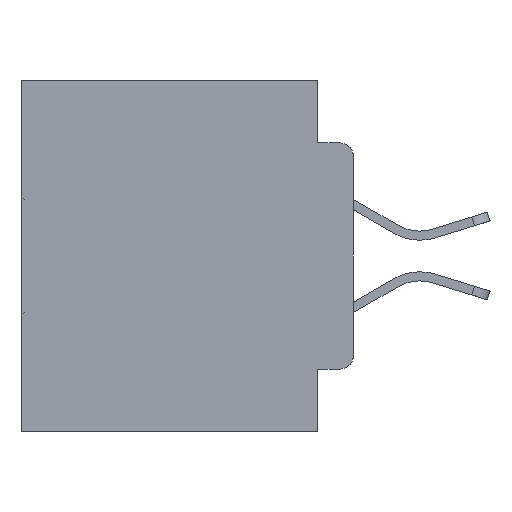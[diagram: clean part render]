
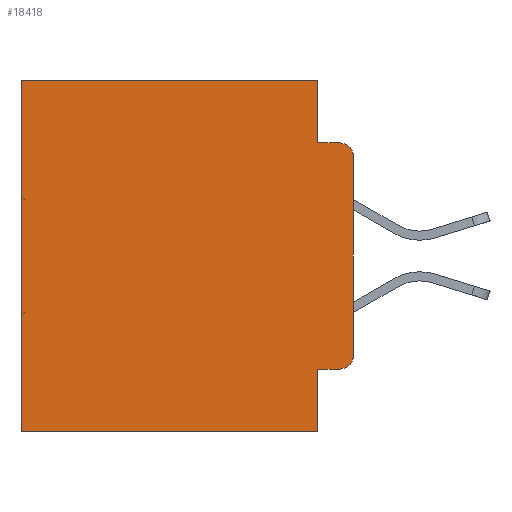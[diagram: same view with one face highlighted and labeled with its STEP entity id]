
A CAD part, left-side view. The second image highlights one B-rep face of the part: STEP entity #18418.
In plain terms, the highlighted planar face has unit normal (-1, 0, 0).
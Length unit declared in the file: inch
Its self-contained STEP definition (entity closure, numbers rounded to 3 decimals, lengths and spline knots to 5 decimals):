
#208 = CARTESIAN_POINT ( 'NONE',  ( 0.298, 0.473, 0. ) ) ;
#493 = CARTESIAN_POINT ( 'NONE',  ( 0.298, 0.051, 0. ) ) ;
#1325 = CARTESIAN_POINT ( 'NONE',  ( 0.298, 0.051, -0.0885 ) ) ;
#1453 = CARTESIAN_POINT ( 'NONE',  ( 0.298, 0.051, 0. ) ) ;
#1546 = VERTEX_POINT ( 'NONE', #14680 ) ;
#1714 = EDGE_CURVE ( 'NONE', #9751, #1546, #14060, .T. ) ;
#2243 = LINE ( 'NONE', #13286, #20582 ) ;
#2251 = LINE ( 'NONE', #27354, #27977 ) ;
#2500 = CARTESIAN_POINT ( 'NONE',  ( 0.298, 0.051, -0.4115 ) ) ;
#2796 = CARTESIAN_POINT ( 'NONE',  ( 0.298, 0.473, -0.5 ) ) ;
#2887 = CARTESIAN_POINT ( 'NONE',  ( 0.298, 0.051, 0. ) ) ;
#3196 = EDGE_CURVE ( 'NONE', #13413, #29406, #16702, .T. ) ;
#3842 = CARTESIAN_POINT ( 'NONE',  ( 0.298, 0.473, 0. ) ) ;
#3933 = DIRECTION ( 'NONE',  ( 0., 0., -1. ) ) ;
#5208 = DIRECTION ( 'NONE',  ( 0., -1., 0. ) ) ;
#7152 = DIRECTION ( 'NONE',  ( -1., 0., 0. ) ) ;
#7243 = VERTEX_POINT ( 'NONE', #1453 ) ;
#7281 = DIRECTION ( 'NONE',  ( 1., 0., 0. ) ) ;
#7400 = DIRECTION ( 'NONE',  ( 0., 0., -1. ) ) ;
#7687 = EDGE_CURVE ( 'NONE', #7243, #22381, #15127, .T. ) ;
#9164 = ORIENTED_EDGE ( 'NONE', *, *, #30143, .T. ) ;
#9751 = VERTEX_POINT ( 'NONE', #31680 ) ;
#10333 = EDGE_CURVE ( 'NONE', #22381, #19065, #28598, .T. ) ;
#13094 = VERTEX_POINT ( 'NONE', #1325 ) ;
#13286 = CARTESIAN_POINT ( 'NONE',  ( 0.298, 0.051, -0.0885 ) ) ;
#13410 = EDGE_CURVE ( 'NONE', #9751, #15226, #2251, .T. ) ;
#13413 = VERTEX_POINT ( 'NONE', #2500 ) ;
#13834 = CARTESIAN_POINT ( 'NONE',  ( 0.298, 0., -0.3915 ) ) ;
#14060 = CIRCLE ( 'NONE', #30863, 0.02 ) ;
#14680 = CARTESIAN_POINT ( 'NONE',  ( 0.298, 0.02, -0.0885 ) ) ;
#15127 = LINE ( 'NONE', #32003, #20955 ) ;
#15196 = FACE_OUTER_BOUND ( 'NONE', #16358, .T. ) ;
#15226 = VERTEX_POINT ( 'NONE', #13834 ) ;
#16358 = EDGE_LOOP ( 'NONE', ( #20195, #21744, #18322, #17511, #27207, #32156, #25284, #31083, #28011, #9164 ) ) ;
#16619 = LINE ( 'NONE', #493, #29809 ) ;
#16702 = LINE ( 'NONE', #17954, #22491 ) ;
#16835 = LINE ( 'NONE', #2887, #22619 ) ;
#17296 = CARTESIAN_POINT ( 'NONE',  ( 0.298, 0., -0.5 ) ) ;
#17442 = EDGE_CURVE ( 'NONE', #13413, #28976, #16835, .T. ) ;
#17511 = ORIENTED_EDGE ( 'NONE', *, *, #27279, .F. ) ;
#17954 = CARTESIAN_POINT ( 'NONE',  ( 0.298, 0.051, -0.4115 ) ) ;
#18322 = ORIENTED_EDGE ( 'NONE', *, *, #26248, .F. ) ;
#18418 = ADVANCED_FACE ( 'NONE', ( #15196 ), #27150, .F. ) ;
#19065 = VERTEX_POINT ( 'NONE', #2796 ) ;
#19642 = CARTESIAN_POINT ( 'NONE',  ( 0.298, 0., 0. ) ) ;
#20195 = ORIENTED_EDGE ( 'NONE', *, *, #13410, .F. ) ;
#20582 = VECTOR ( 'NONE', #23174, 39.37008 ) ;
#20920 = AXIS2_PLACEMENT_3D ( 'NONE', #19642, #7281, #24743 ) ;
#20955 = VECTOR ( 'NONE', #21054, 39.37008 ) ;
#21054 = DIRECTION ( 'NONE',  ( 0., 1., 0. ) ) ;
#21621 = EDGE_CURVE ( 'NONE', #28976, #19065, #28153, .T. ) ;
#21744 = ORIENTED_EDGE ( 'NONE', *, *, #1714, .T. ) ;
#21951 = VECTOR ( 'NONE', #3933, 39.37008 ) ;
#22078 = CARTESIAN_POINT ( 'NONE',  ( 0.298, 0.02, -0.3915 ) ) ;
#22274 = VECTOR ( 'NONE', #32058, 39.37008 ) ;
#22381 = VERTEX_POINT ( 'NONE', #208 ) ;
#22487 = CARTESIAN_POINT ( 'NONE',  ( 0.298, 0.051, -0.5 ) ) ;
#22491 = VECTOR ( 'NONE', #5208, 39.37008 ) ;
#22619 = VECTOR ( 'NONE', #22825, 39.37008 ) ;
#22825 = DIRECTION ( 'NONE',  ( 0., 0., -1. ) ) ;
#23174 = DIRECTION ( 'NONE',  ( 0., -1., 0. ) ) ;
#23420 = CIRCLE ( 'NONE', #32046, 0.02 ) ;
#24620 = DIRECTION ( 'NONE',  ( 0., 0., -1. ) ) ;
#24743 = DIRECTION ( 'NONE',  ( 0., 0., -1. ) ) ;
#25284 = ORIENTED_EDGE ( 'NONE', *, *, #21621, .F. ) ;
#25457 = DIRECTION ( 'NONE',  ( 0., 0., -1. ) ) ;
#26061 = DIRECTION ( 'NONE',  ( -1., 0., 0. ) ) ;
#26248 = EDGE_CURVE ( 'NONE', #13094, #1546, #2243, .T. ) ;
#26312 = CARTESIAN_POINT ( 'NONE',  ( 0.298, 0.02, -0.4115 ) ) ;
#27150 = PLANE ( 'NONE',  #20920 ) ;
#27207 = ORIENTED_EDGE ( 'NONE', *, *, #7687, .T. ) ;
#27279 = EDGE_CURVE ( 'NONE', #7243, #13094, #16619, .T. ) ;
#27354 = CARTESIAN_POINT ( 'NONE',  ( 0.298, 0., 0. ) ) ;
#27977 = VECTOR ( 'NONE', #7400, 39.37008 ) ;
#28011 = ORIENTED_EDGE ( 'NONE', *, *, #3196, .T. ) ;
#28153 = LINE ( 'NONE', #17296, #22274 ) ;
#28598 = LINE ( 'NONE', #3842, #21951 ) ;
#28976 = VERTEX_POINT ( 'NONE', #22487 ) ;
#29300 = DIRECTION ( 'NONE',  ( 0., 0., -1. ) ) ;
#29406 = VERTEX_POINT ( 'NONE', #26312 ) ;
#29809 = VECTOR ( 'NONE', #25457, 39.37008 ) ;
#30143 = EDGE_CURVE ( 'NONE', #29406, #15226, #23420, .T. ) ;
#30863 = AXIS2_PLACEMENT_3D ( 'NONE', #31838, #26061, #29300 ) ;
#31083 = ORIENTED_EDGE ( 'NONE', *, *, #17442, .F. ) ;
#31680 = CARTESIAN_POINT ( 'NONE',  ( 0.298, 0., -0.1085 ) ) ;
#31838 = CARTESIAN_POINT ( 'NONE',  ( 0.298, 0.02, -0.1085 ) ) ;
#32003 = CARTESIAN_POINT ( 'NONE',  ( 0.298, 0., 0. ) ) ;
#32046 = AXIS2_PLACEMENT_3D ( 'NONE', #22078, #7152, #24620 ) ;
#32058 = DIRECTION ( 'NONE',  ( 0., 1., 0. ) ) ;
#32156 = ORIENTED_EDGE ( 'NONE', *, *, #10333, .T. ) ;
